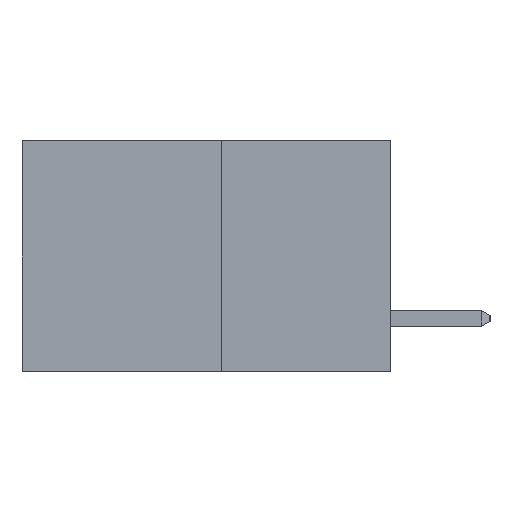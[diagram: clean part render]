
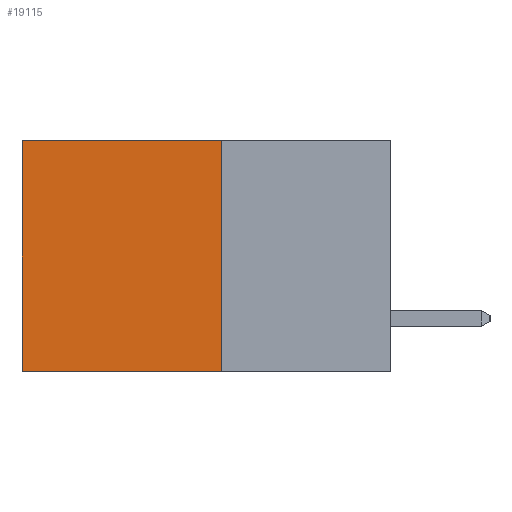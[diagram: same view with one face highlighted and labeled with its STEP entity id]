
A CAD part, left-side view. The second image highlights one B-rep face of the part: STEP entity #19115.
In plain terms, the highlighted planar face has unit normal (-1, 0, 0).
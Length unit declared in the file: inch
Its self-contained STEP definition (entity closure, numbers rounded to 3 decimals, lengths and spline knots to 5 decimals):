
#1201 = VECTOR ( 'NONE', #18981, 39.37008 ) ;
#1306 = EDGE_CURVE ( 'NONE', #5784, #3359, #23348, .T. ) ;
#1525 = CARTESIAN_POINT ( 'NONE',  ( 0.277, 0.27, -0.37 ) ) ;
#2305 = CARTESIAN_POINT ( 'NONE',  ( 0.277, 0.27, -0.37 ) ) ;
#2765 = VECTOR ( 'NONE', #14641, 39.37008 ) ;
#3300 = CARTESIAN_POINT ( 'NONE',  ( 0.277, 0.59, -0.37 ) ) ;
#3359 = VERTEX_POINT ( 'NONE', #3300 ) ;
#3399 = DIRECTION ( 'NONE',  ( 0., 0., -1. ) ) ;
#3479 = VECTOR ( 'NONE', #17134, 39.37008 ) ;
#4398 = EDGE_CURVE ( 'NONE', #6082, #3359, #6144, .T. ) ;
#4809 = ORIENTED_EDGE ( 'NONE', *, *, #13263, .F. ) ;
#5092 = CARTESIAN_POINT ( 'NONE',  ( 0.277, 0.59, 0. ) ) ;
#5428 = ORIENTED_EDGE ( 'NONE', *, *, #1306, .F. ) ;
#5784 = VERTEX_POINT ( 'NONE', #2305 ) ;
#6065 = FACE_OUTER_BOUND ( 'NONE', #13562, .T. ) ;
#6082 = VERTEX_POINT ( 'NONE', #5092 ) ;
#6144 = LINE ( 'NONE', #11643, #1201 ) ;
#11132 = DIRECTION ( 'NONE',  ( 0., 1., 0. ) ) ;
#11150 = EDGE_CURVE ( 'NONE', #11551, #6082, #16630, .T. ) ;
#11551 = VERTEX_POINT ( 'NONE', #17364 ) ;
#11643 = CARTESIAN_POINT ( 'NONE',  ( 0.277, 0.59, -0.37 ) ) ;
#12932 = CARTESIAN_POINT ( 'NONE',  ( 0.277, 0.27, 0. ) ) ;
#13263 = EDGE_CURVE ( 'NONE', #11551, #5784, #13347, .T. ) ;
#13347 = LINE ( 'NONE', #15287, #3479 ) ;
#13562 = EDGE_LOOP ( 'NONE', ( #23113, #5428, #4809, #20668 ) ) ;
#13610 = CARTESIAN_POINT ( 'NONE',  ( 0.277, 0.27, -0.37 ) ) ;
#14500 = DIRECTION ( 'NONE',  ( 1., 0., 0. ) ) ;
#14641 = DIRECTION ( 'NONE',  ( 0., 1., 0. ) ) ;
#15287 = CARTESIAN_POINT ( 'NONE',  ( 0.277, 0.27, -0.37 ) ) ;
#16630 = LINE ( 'NONE', #12932, #20908 ) ;
#17134 = DIRECTION ( 'NONE',  ( 0., 0., -1. ) ) ;
#17364 = CARTESIAN_POINT ( 'NONE',  ( 0.277, 0.27, 0. ) ) ;
#18981 = DIRECTION ( 'NONE',  ( 0., 0., -1. ) ) ;
#19115 = ADVANCED_FACE ( 'NONE', ( #6065 ), #19926, .F. ) ;
#19926 = PLANE ( 'NONE',  #23001 ) ;
#20668 = ORIENTED_EDGE ( 'NONE', *, *, #11150, .T. ) ;
#20908 = VECTOR ( 'NONE', #11132, 39.37008 ) ;
#23001 = AXIS2_PLACEMENT_3D ( 'NONE', #1525, #14500, #3399 ) ;
#23113 = ORIENTED_EDGE ( 'NONE', *, *, #4398, .T. ) ;
#23348 = LINE ( 'NONE', #13610, #2765 ) ;
